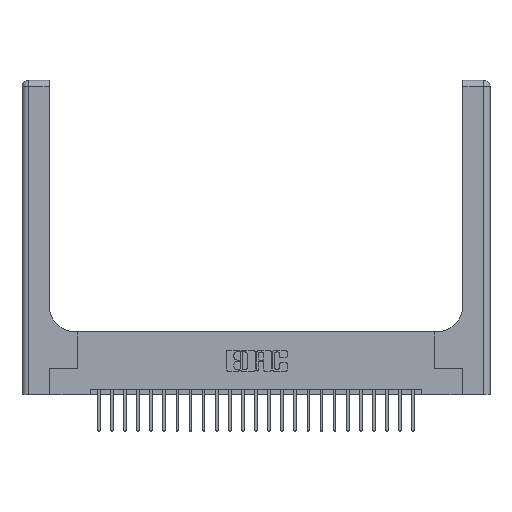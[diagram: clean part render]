
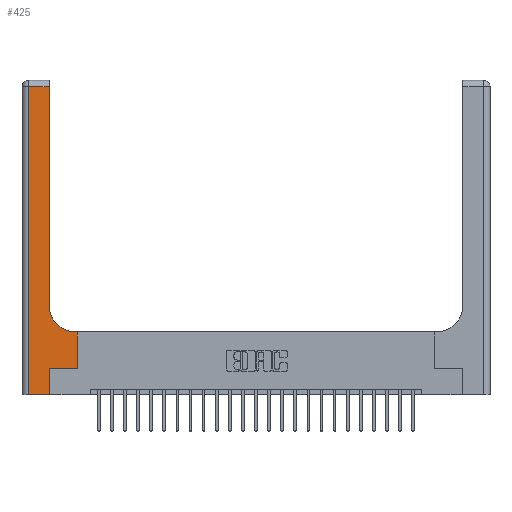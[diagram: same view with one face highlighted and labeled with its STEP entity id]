
A CAD part, top view. The second image highlights one B-rep face of the part: STEP entity #425.
In plain terms, the highlighted planar face has unit normal (0, 0, 1).
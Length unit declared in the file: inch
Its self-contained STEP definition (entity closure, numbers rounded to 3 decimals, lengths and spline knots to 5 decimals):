
#425 = ADVANCED_FACE ( 'NONE', ( #666 ), #18957, .F. ) ;
#455 = VERTEX_POINT ( 'NONE', #21429 ) ;
#609 = ORIENTED_EDGE ( 'NONE', *, *, #22309, .T. ) ;
#666 = FACE_OUTER_BOUND ( 'NONE', #3324, .T. ) ;
#674 = VERTEX_POINT ( 'NONE', #9688 ) ;
#689 = CARTESIAN_POINT ( 'NONE',  ( 0., 3., 0.37 ) ) ;
#1267 = VERTEX_POINT ( 'NONE', #3471 ) ;
#1943 = LINE ( 'NONE', #14903, #6223 ) ;
#3324 = EDGE_LOOP ( 'NONE', ( #6877, #609, #9021, #23103, #13035, #12602, #22679, #13675, #19265 ) ) ;
#3471 = CARTESIAN_POINT ( 'NONE',  ( 0.26, 2.94, 0.37 ) ) ;
#3487 = CIRCLE ( 'NONE', #13238, 0.25 ) ;
#3619 = VERTEX_POINT ( 'NONE', #14723 ) ;
#3876 = LINE ( 'NONE', #9494, #15682 ) ;
#4199 = VECTOR ( 'NONE', #21339, 39.37008 ) ;
#5114 = VECTOR ( 'NONE', #10542, 39.37008 ) ;
#5872 = DIRECTION ( 'NONE',  ( -1., 0., 0. ) ) ;
#5959 = VECTOR ( 'NONE', #23410, 39.37008 ) ;
#6223 = VECTOR ( 'NONE', #20385, 39.37008 ) ;
#6227 = CARTESIAN_POINT ( 'NONE',  ( 0.265, 0.25, 0.37 ) ) ;
#6256 = LINE ( 'NONE', #10300, #5114 ) ;
#6877 = ORIENTED_EDGE ( 'NONE', *, *, #9133, .T. ) ;
#7018 = LINE ( 'NONE', #20526, #11280 ) ;
#7246 = CARTESIAN_POINT ( 'NONE',  ( 0.51, 0.85, 0.37 ) ) ;
#7587 = DIRECTION ( 'NONE',  ( -1., 0., 0. ) ) ;
#8338 = EDGE_CURVE ( 'NONE', #23597, #3619, #10857, .T. ) ;
#9021 = ORIENTED_EDGE ( 'NONE', *, *, #10908, .T. ) ;
#9102 = CARTESIAN_POINT ( 'NONE',  ( 0.528, 0.6, 0.37 ) ) ;
#9133 = EDGE_CURVE ( 'NONE', #674, #1267, #1943, .T. ) ;
#9494 = CARTESIAN_POINT ( 'NONE',  ( 0., 2.94, 0.37 ) ) ;
#9688 = CARTESIAN_POINT ( 'NONE',  ( 0.26, 0.85, 0.37 ) ) ;
#9767 = CARTESIAN_POINT ( 'NONE',  ( 0.06, 2.94, 0.37 ) ) ;
#10064 = CARTESIAN_POINT ( 'NONE',  ( 0., 0., 0.37 ) ) ;
#10275 = VERTEX_POINT ( 'NONE', #6227 ) ;
#10300 = CARTESIAN_POINT ( 'NONE',  ( 0.265, 0., 0.37 ) ) ;
#10379 = DIRECTION ( 'NONE',  ( -1., 0., 0. ) ) ;
#10542 = DIRECTION ( 'NONE',  ( 0., 1., 0. ) ) ;
#10857 = LINE ( 'NONE', #10064, #4199 ) ;
#10908 = EDGE_CURVE ( 'NONE', #18311, #23597, #17393, .T. ) ;
#11280 = VECTOR ( 'NONE', #7587, 39.37008 ) ;
#11830 = EDGE_CURVE ( 'NONE', #18033, #19128, #7018, .T. ) ;
#11913 = DIRECTION ( 'NONE',  ( 0., 1., 0. ) ) ;
#12278 = LINE ( 'NONE', #23327, #5959 ) ;
#12602 = ORIENTED_EDGE ( 'NONE', *, *, #16009, .T. ) ;
#12871 = VECTOR ( 'NONE', #11913, 39.37008 ) ;
#13035 = ORIENTED_EDGE ( 'NONE', *, *, #14682, .T. ) ;
#13205 = EDGE_CURVE ( 'NONE', #19128, #674, #3487, .T. ) ;
#13238 = AXIS2_PLACEMENT_3D ( 'NONE', #7246, #20111, #18458 ) ;
#13675 = ORIENTED_EDGE ( 'NONE', *, *, #11830, .T. ) ;
#14143 = CARTESIAN_POINT ( 'NONE',  ( 0.06, 3., 0.37 ) ) ;
#14682 = EDGE_CURVE ( 'NONE', #3619, #10275, #6256, .T. ) ;
#14723 = CARTESIAN_POINT ( 'NONE',  ( 0.265, 0., 0.37 ) ) ;
#14903 = CARTESIAN_POINT ( 'NONE',  ( 0.26, 3., 0.37 ) ) ;
#14942 = EDGE_CURVE ( 'NONE', #455, #18033, #21249, .T. ) ;
#15682 = VECTOR ( 'NONE', #5872, 39.37008 ) ;
#16009 = EDGE_CURVE ( 'NONE', #10275, #455, #12278, .T. ) ;
#16117 = CARTESIAN_POINT ( 'NONE',  ( 0.51, 0.6, 0.37 ) ) ;
#16819 = VECTOR ( 'NONE', #21566, 39.37008 ) ;
#17320 = CARTESIAN_POINT ( 'NONE',  ( 0.06, 0., 0.37 ) ) ;
#17393 = LINE ( 'NONE', #14143, #16819 ) ;
#17414 = CARTESIAN_POINT ( 'NONE',  ( 0.528, 0.25, 0.37 ) ) ;
#18033 = VERTEX_POINT ( 'NONE', #9102 ) ;
#18311 = VERTEX_POINT ( 'NONE', #9767 ) ;
#18458 = DIRECTION ( 'NONE',  ( 1., 0., 0. ) ) ;
#18957 = PLANE ( 'NONE',  #21255 ) ;
#19121 = DIRECTION ( 'NONE',  ( 0., 0., -1. ) ) ;
#19128 = VERTEX_POINT ( 'NONE', #16117 ) ;
#19265 = ORIENTED_EDGE ( 'NONE', *, *, #13205, .T. ) ;
#20111 = DIRECTION ( 'NONE',  ( 0., 0., -1. ) ) ;
#20385 = DIRECTION ( 'NONE',  ( 0., 1., 0. ) ) ;
#20526 = CARTESIAN_POINT ( 'NONE',  ( 0.26, 0.6, 0.37 ) ) ;
#21249 = LINE ( 'NONE', #17414, #12871 ) ;
#21255 = AXIS2_PLACEMENT_3D ( 'NONE', #689, #19121, #10379 ) ;
#21339 = DIRECTION ( 'NONE',  ( 1., 0., 0. ) ) ;
#21429 = CARTESIAN_POINT ( 'NONE',  ( 0.528, 0.25, 0.37 ) ) ;
#21566 = DIRECTION ( 'NONE',  ( 0., -1., 0. ) ) ;
#22309 = EDGE_CURVE ( 'NONE', #1267, #18311, #3876, .T. ) ;
#22679 = ORIENTED_EDGE ( 'NONE', *, *, #14942, .T. ) ;
#23103 = ORIENTED_EDGE ( 'NONE', *, *, #8338, .T. ) ;
#23327 = CARTESIAN_POINT ( 'NONE',  ( 0.265, 0.25, 0.37 ) ) ;
#23410 = DIRECTION ( 'NONE',  ( 1., 0., 0. ) ) ;
#23597 = VERTEX_POINT ( 'NONE', #17320 ) ;
